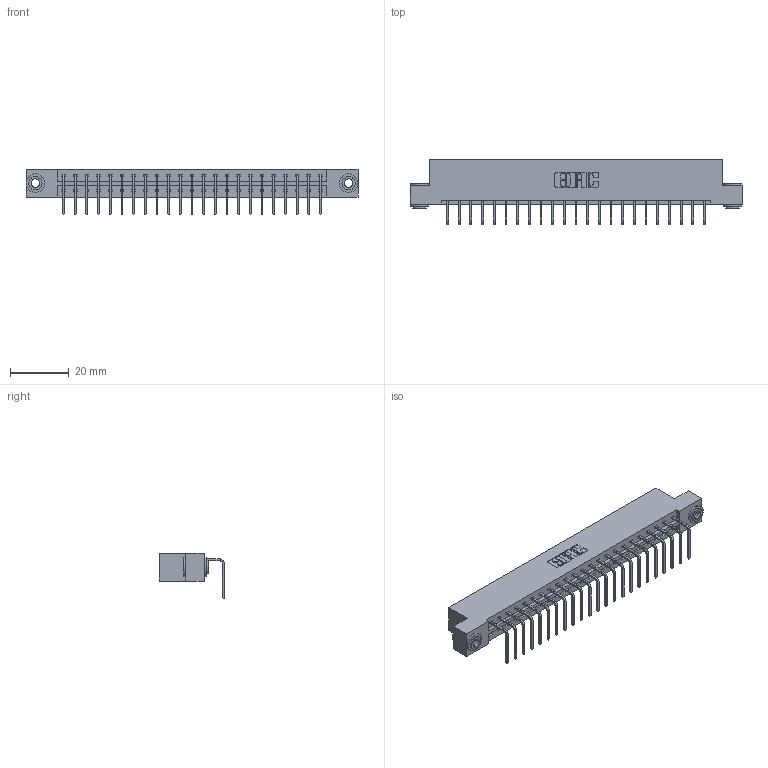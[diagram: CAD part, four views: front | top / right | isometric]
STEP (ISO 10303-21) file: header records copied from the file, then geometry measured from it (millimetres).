
FILE_DESCRIPTION (( 'STEP AP203' ), '1' );
FILE_NAME ('833-023-558-103.STEP', '2020-06-01T19:38:45', ( '' ), ( '' ), 'SwSTEP 2.0', 'SolidWorks 2020', '' );
FILE_SCHEMA (( 'CONFIG_CONTROL_DESIGN' ));
Length unit declared in the file: inch
Products named in the file (4): 345-292-001_558 Tail - 2; 833 Part_Flush - .156 Dia - TH; 345-250-002_345-250-002-102; 833-023-558-103
Assembly tree (26 placements, depth 2):
  833-023-558-103
    833 Part_Flush - .156 Dia - TH
    345-292-001_558 Tail - 2  x23
    345-250-002_345-250-002-102  x2
Bounding box: 112.67 x 22.17 x 15.37 mm (x, y, z)
Volume: 11270.8 mm3; surface area: 12768 mm2
Topology: 26 solids, 26 shells, 1532 faces, 4573 edges, 3014 vertices
Faces by surface type: plane 1092, cylinder 432, cone 8
Entity records: 17252 total; most frequent: CARTESIAN_POINT 2958, ORIENTED_EDGE 2910, DIRECTION 2567, EDGE_CURVE 1455, LINE 1303, VECTOR 1303, VERTEX_POINT 966, AXIS2_PLACEMENT_3D 632
